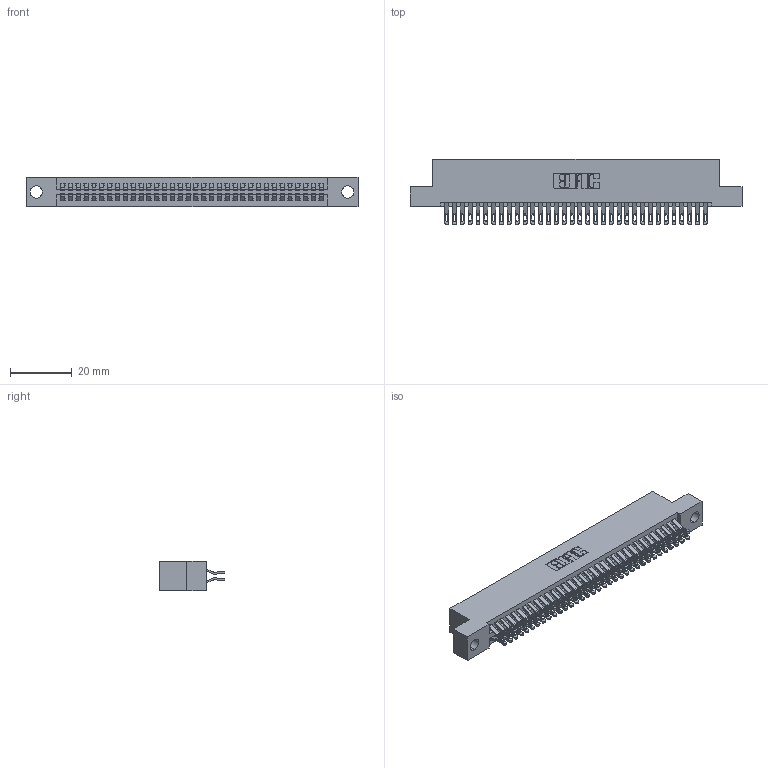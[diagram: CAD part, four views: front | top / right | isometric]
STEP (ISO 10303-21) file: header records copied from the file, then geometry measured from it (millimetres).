
FILE_DESCRIPTION (( 'STEP AP203' ), '1' );
FILE_NAME ('395-068-555-204.STEP', '2018-11-25T18:34:13', ( '' ), ( '' ), 'SwSTEP 2.0', 'SolidWorks 2016', '' );
FILE_SCHEMA (( 'CONFIG_CONTROL_DESIGN' ));
Length unit declared in the file: inch
Products named in the file (3): 395-068-555-204; 345 Part_Flush Mounting Lugs - 0.156 Dia-TH; 345-292-001_555 Tail
Assembly tree (69 placements, depth 2):
  395-068-555-204
    345 Part_Flush Mounting Lugs - 0.156 Dia-TH
    345-292-001_555 Tail  x68
Bounding box: 107.57 x 21.13 x 9.4 mm (x, y, z)
Volume: 10484.5 mm3; surface area: 15844.1 mm2
Topology: 69 solids, 69 shells, 3934 faces, 12377 edges, 8250 vertices
Faces by surface type: plane 2188, cylinder 1746
Entity records: 28083 total; most frequent: CARTESIAN_POINT 4750, ORIENTED_EDGE 4654, DIRECTION 4167, EDGE_CURVE 2327, LINE 2039, VECTOR 2039, VERTEX_POINT 1550, AXIS2_PLACEMENT_3D 1064
